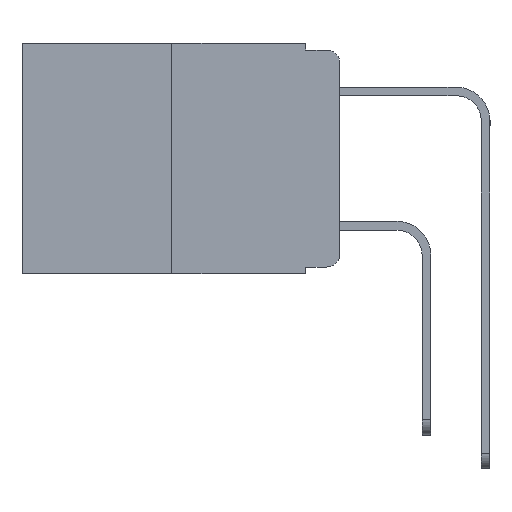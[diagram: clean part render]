
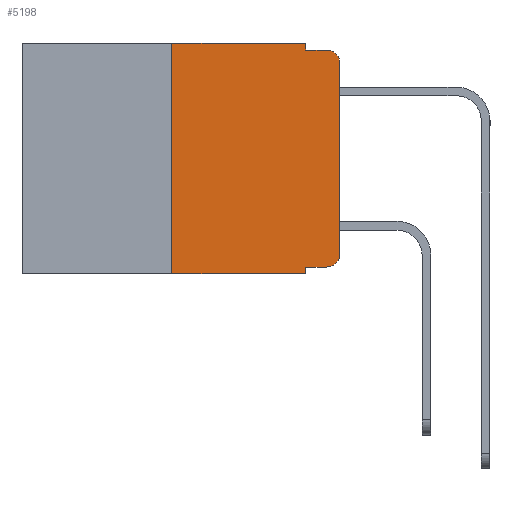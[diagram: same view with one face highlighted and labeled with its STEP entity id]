
A CAD part, left-side view. The second image highlights one B-rep face of the part: STEP entity #5198.
In plain terms, the highlighted planar face has unit normal (-1, 0, 0).
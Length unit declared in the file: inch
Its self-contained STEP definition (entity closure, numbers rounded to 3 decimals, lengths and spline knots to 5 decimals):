
#20 = EDGE_CURVE ( 'NONE', #2411, #12989, #3648, .T. ) ;
#52 = FACE_OUTER_BOUND ( 'NONE', #12680, .T. ) ;
#327 = DIRECTION ( 'NONE',  ( 0., 0., -1. ) ) ;
#1273 = DIRECTION ( 'NONE',  ( 0., -1., 0. ) ) ;
#1642 = VERTEX_POINT ( 'NONE', #4198 ) ;
#1814 = VECTOR ( 'NONE', #5721, 39.37008 ) ;
#2093 = PLANE ( 'NONE',  #4983 ) ;
#2114 = VERTEX_POINT ( 'NONE', #3827 ) ;
#2235 = CARTESIAN_POINT ( 'NONE',  ( 0., 0.25, -0.343 ) ) ;
#2411 = VERTEX_POINT ( 'NONE', #2235 ) ;
#2581 = EDGE_CURVE ( 'NONE', #2114, #4788, #15069, .T. ) ;
#2832 = VECTOR ( 'NONE', #11058, 39.37008 ) ;
#2877 = CARTESIAN_POINT ( 'NONE',  ( 0., 0.051, 0. ) ) ;
#2887 = EDGE_CURVE ( 'NONE', #1642, #8074, #11146, .T. ) ;
#2906 = AXIS2_PLACEMENT_3D ( 'NONE', #12278, #12275, #12258 ) ;
#3298 = VECTOR ( 'NONE', #4798, 39.37008 ) ;
#3391 = CARTESIAN_POINT ( 'NONE',  ( 0., 0., -0.03 ) ) ;
#3648 = LINE ( 'NONE', #5720, #3298 ) ;
#3749 = ORIENTED_EDGE ( 'NONE', *, *, #4929, .F. ) ;
#3827 = CARTESIAN_POINT ( 'NONE',  ( 0., 0.02, -0.333 ) ) ;
#4014 = CARTESIAN_POINT ( 'NONE',  ( 0., 0.051, -0.333 ) ) ;
#4142 = EDGE_CURVE ( 'NONE', #10489, #2114, #14495, .T. ) ;
#4198 = CARTESIAN_POINT ( 'NONE',  ( 0., 0.25, 0. ) ) ;
#4250 = DIRECTION ( 'NONE',  ( 1., 0., 0. ) ) ;
#4295 = CARTESIAN_POINT ( 'NONE',  ( 0., 0.02, -0.01 ) ) ;
#4315 = LINE ( 'NONE', #10385, #7043 ) ;
#4365 = CARTESIAN_POINT ( 'NONE',  ( 0., 0., 0. ) ) ;
#4502 = VECTOR ( 'NONE', #11348, 39.37008 ) ;
#4533 = AXIS2_PLACEMENT_3D ( 'NONE', #14335, #7394, #327 ) ;
#4788 = VERTEX_POINT ( 'NONE', #11747 ) ;
#4798 = DIRECTION ( 'NONE',  ( 0., -1., 0. ) ) ;
#4929 = EDGE_CURVE ( 'NONE', #10489, #12989, #4315, .T. ) ;
#4983 = AXIS2_PLACEMENT_3D ( 'NONE', #5855, #4250, #12420 ) ;
#5198 = ADVANCED_FACE ( 'NONE', ( #52 ), #2093, .F. ) ;
#5203 = ORIENTED_EDGE ( 'NONE', *, *, #6490, .F. ) ;
#5268 = VECTOR ( 'NONE', #5534, 39.37008 ) ;
#5495 = ORIENTED_EDGE ( 'NONE', *, *, #10423, .T. ) ;
#5534 = DIRECTION ( 'NONE',  ( 0., 0., 1. ) ) ;
#5720 = CARTESIAN_POINT ( 'NONE',  ( 0., 0.473, -0.343 ) ) ;
#5721 = DIRECTION ( 'NONE',  ( 0., -1., 0. ) ) ;
#5746 = ORIENTED_EDGE ( 'NONE', *, *, #7268, .F. ) ;
#5855 = CARTESIAN_POINT ( 'NONE',  ( 0., 0.473, 0. ) ) ;
#5868 = DIRECTION ( 'NONE',  ( 0., 0., -1. ) ) ;
#5931 = LINE ( 'NONE', #2877, #2832 ) ;
#5939 = CARTESIAN_POINT ( 'NONE',  ( 0., 0.051, -0.01 ) ) ;
#6132 = ORIENTED_EDGE ( 'NONE', *, *, #2581, .T. ) ;
#6490 = EDGE_CURVE ( 'NONE', #2411, #1642, #11093, .T. ) ;
#6881 = CARTESIAN_POINT ( 'NONE',  ( 0., 0.051, 0. ) ) ;
#7043 = VECTOR ( 'NONE', #5868, 39.37008 ) ;
#7268 = EDGE_CURVE ( 'NONE', #8074, #12099, #5931, .T. ) ;
#7394 = DIRECTION ( 'NONE',  ( -1., 0., 0. ) ) ;
#7525 = VERTEX_POINT ( 'NONE', #3391 ) ;
#7940 = ORIENTED_EDGE ( 'NONE', *, *, #2887, .F. ) ;
#7979 = DIRECTION ( 'NONE',  ( 0., -1., 0. ) ) ;
#8074 = VERTEX_POINT ( 'NONE', #6881 ) ;
#8244 = VECTOR ( 'NONE', #1273, 39.37008 ) ;
#8352 = VECTOR ( 'NONE', #7979, 39.37008 ) ;
#8779 = CARTESIAN_POINT ( 'NONE',  ( 0., 0.25, 0. ) ) ;
#8849 = EDGE_CURVE ( 'NONE', #12099, #11028, #11375, .T. ) ;
#8913 = CARTESIAN_POINT ( 'NONE',  ( 0., 0.051, -0.343 ) ) ;
#9433 = ORIENTED_EDGE ( 'NONE', *, *, #20, .T. ) ;
#9635 = EDGE_CURVE ( 'NONE', #7525, #11028, #10427, .T. ) ;
#9715 = ORIENTED_EDGE ( 'NONE', *, *, #9635, .T. ) ;
#9961 = CARTESIAN_POINT ( 'NONE',  ( 0., 0.051, -0.01 ) ) ;
#10385 = CARTESIAN_POINT ( 'NONE',  ( 0., 0.051, 0. ) ) ;
#10423 = EDGE_CURVE ( 'NONE', #4788, #7525, #11853, .T. ) ;
#10427 = CIRCLE ( 'NONE', #4533, 0.02 ) ;
#10489 = VERTEX_POINT ( 'NONE', #11475 ) ;
#11028 = VERTEX_POINT ( 'NONE', #4295 ) ;
#11058 = DIRECTION ( 'NONE',  ( 0., 0., -1. ) ) ;
#11093 = LINE ( 'NONE', #8779, #4502 ) ;
#11146 = LINE ( 'NONE', #11987, #1814 ) ;
#11348 = DIRECTION ( 'NONE',  ( 0., 0., 1. ) ) ;
#11375 = LINE ( 'NONE', #5939, #8244 ) ;
#11475 = CARTESIAN_POINT ( 'NONE',  ( 0., 0.051, -0.333 ) ) ;
#11562 = ORIENTED_EDGE ( 'NONE', *, *, #8849, .F. ) ;
#11747 = CARTESIAN_POINT ( 'NONE',  ( 0., 0., -0.313 ) ) ;
#11853 = LINE ( 'NONE', #4365, #5268 ) ;
#11987 = CARTESIAN_POINT ( 'NONE',  ( 0., 0.473, 0. ) ) ;
#12099 = VERTEX_POINT ( 'NONE', #9961 ) ;
#12258 = DIRECTION ( 'NONE',  ( 0., 0., -1. ) ) ;
#12275 = DIRECTION ( 'NONE',  ( -1., 0., 0. ) ) ;
#12278 = CARTESIAN_POINT ( 'NONE',  ( 0., 0.02, -0.313 ) ) ;
#12420 = DIRECTION ( 'NONE',  ( 0., 0., -1. ) ) ;
#12680 = EDGE_LOOP ( 'NONE', ( #5495, #9715, #11562, #5746, #7940, #5203, #9433, #3749, #14121, #6132 ) ) ;
#12989 = VERTEX_POINT ( 'NONE', #8913 ) ;
#14121 = ORIENTED_EDGE ( 'NONE', *, *, #4142, .T. ) ;
#14335 = CARTESIAN_POINT ( 'NONE',  ( 0., 0.02, -0.03 ) ) ;
#14495 = LINE ( 'NONE', #4014, #8352 ) ;
#15069 = CIRCLE ( 'NONE', #2906, 0.02 ) ;
